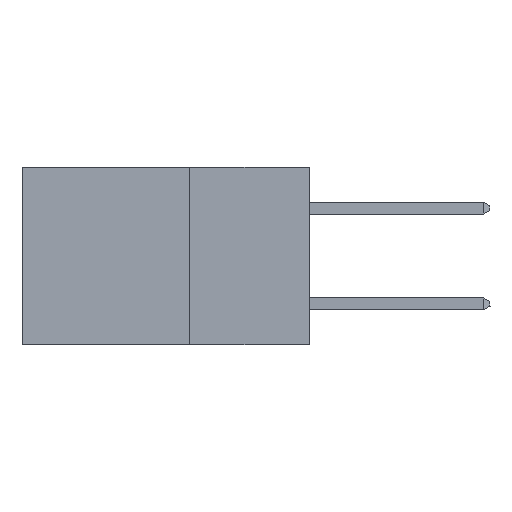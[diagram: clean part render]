
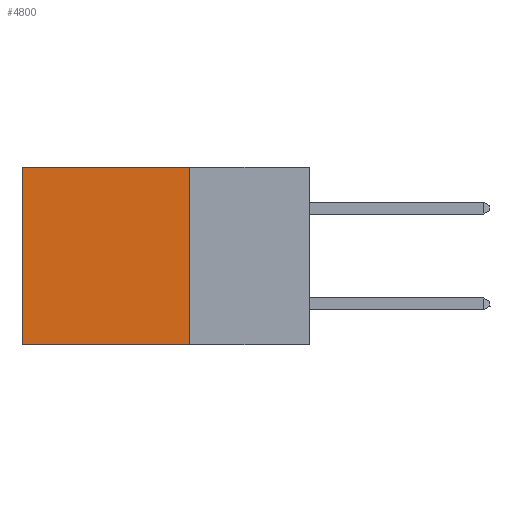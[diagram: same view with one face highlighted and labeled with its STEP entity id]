
A CAD part, left-side view. The second image highlights one B-rep face of the part: STEP entity #4800.
In plain terms, the highlighted planar face has unit normal (-1, 0, 0).
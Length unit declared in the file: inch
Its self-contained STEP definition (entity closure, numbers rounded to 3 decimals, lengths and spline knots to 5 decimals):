
#62 = LINE ( 'NONE', #12425, #545 ) ;
#351 = EDGE_CURVE ( 'NONE', #14972, #5731, #6886, .T. ) ;
#516 = CARTESIAN_POINT ( 'NONE',  ( 0.2875, 0.6, -0.37 ) ) ;
#545 = VECTOR ( 'NONE', #17644, 39.37008 ) ;
#1506 = CARTESIAN_POINT ( 'NONE',  ( 0.2875, 0.25, -0.37 ) ) ;
#1785 = DIRECTION ( 'NONE',  ( 1., 0., 0. ) ) ;
#1994 = VECTOR ( 'NONE', #15715, 39.37008 ) ;
#3124 = AXIS2_PLACEMENT_3D ( 'NONE', #5402, #1785, #7276 ) ;
#3291 = ORIENTED_EDGE ( 'NONE', *, *, #5603, .T. ) ;
#3418 = PLANE ( 'NONE',  #3124 ) ;
#3708 = EDGE_LOOP ( 'NONE', ( #3291, #4274, #21727, #9865 ) ) ;
#4274 = ORIENTED_EDGE ( 'NONE', *, *, #351, .F. ) ;
#4800 = ADVANCED_FACE ( 'NONE', ( #8682 ), #3418, .F. ) ;
#5136 = LINE ( 'NONE', #17350, #9596 ) ;
#5402 = CARTESIAN_POINT ( 'NONE',  ( 0.2875, 0.25, 0. ) ) ;
#5603 = EDGE_CURVE ( 'NONE', #20810, #5731, #62, .T. ) ;
#5731 = VERTEX_POINT ( 'NONE', #516 ) ;
#6886 = LINE ( 'NONE', #1506, #1994 ) ;
#7276 = DIRECTION ( 'NONE',  ( 0., 0., -1. ) ) ;
#8215 = DIRECTION ( 'NONE',  ( 0., 0., -1. ) ) ;
#8643 = CARTESIAN_POINT ( 'NONE',  ( 0.2875, 0.6, 0. ) ) ;
#8682 = FACE_OUTER_BOUND ( 'NONE', #3708, .T. ) ;
#9596 = VECTOR ( 'NONE', #20838, 39.37008 ) ;
#9865 = ORIENTED_EDGE ( 'NONE', *, *, #22161, .T. ) ;
#12425 = CARTESIAN_POINT ( 'NONE',  ( 0.2875, 0.6, 0. ) ) ;
#13446 = CARTESIAN_POINT ( 'NONE',  ( 0.2875, 0.25, 0. ) ) ;
#14452 = CARTESIAN_POINT ( 'NONE',  ( 0.2875, 0.25, 0. ) ) ;
#14972 = VERTEX_POINT ( 'NONE', #17587 ) ;
#15149 = VERTEX_POINT ( 'NONE', #14452 ) ;
#15715 = DIRECTION ( 'NONE',  ( 0., 1., 0. ) ) ;
#16954 = VECTOR ( 'NONE', #8215, 39.37008 ) ;
#17350 = CARTESIAN_POINT ( 'NONE',  ( 0.2875, 0.25, 0. ) ) ;
#17587 = CARTESIAN_POINT ( 'NONE',  ( 0.2875, 0.25, -0.37 ) ) ;
#17644 = DIRECTION ( 'NONE',  ( 0., 0., -1. ) ) ;
#20283 = EDGE_CURVE ( 'NONE', #15149, #14972, #20418, .T. ) ;
#20418 = LINE ( 'NONE', #13446, #16954 ) ;
#20810 = VERTEX_POINT ( 'NONE', #8643 ) ;
#20838 = DIRECTION ( 'NONE',  ( 0., 1., 0. ) ) ;
#21727 = ORIENTED_EDGE ( 'NONE', *, *, #20283, .F. ) ;
#22161 = EDGE_CURVE ( 'NONE', #15149, #20810, #5136, .T. ) ;
